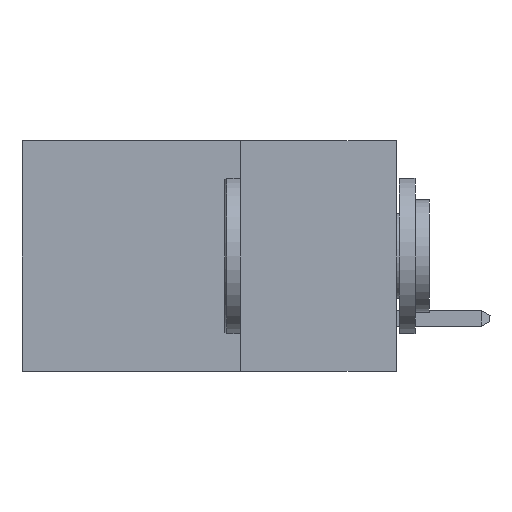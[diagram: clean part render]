
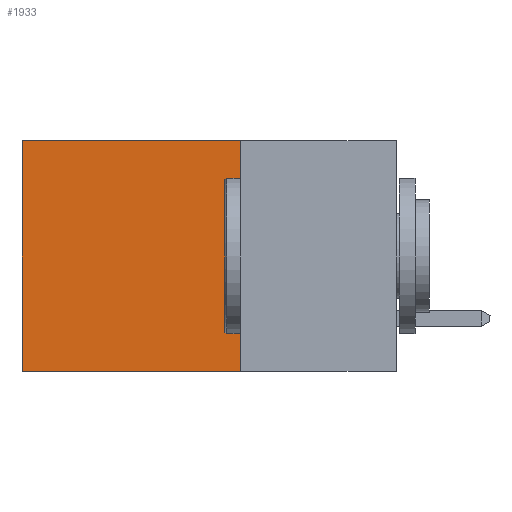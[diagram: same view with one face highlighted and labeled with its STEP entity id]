
A CAD part, left-side view. The second image highlights one B-rep face of the part: STEP entity #1933.
In plain terms, the highlighted planar face has unit normal (-1, 0, 0).
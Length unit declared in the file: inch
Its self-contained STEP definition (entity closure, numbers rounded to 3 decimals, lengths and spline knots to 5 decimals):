
#49 = ORIENTED_EDGE ( 'NONE', *, *, #5225, .F. ) ;
#374 = CARTESIAN_POINT ( 'NONE',  ( 0.2615, 0.25, -0.37 ) ) ;
#1356 = EDGE_CURVE ( 'NONE', #13783, #1747, #13322, .T. ) ;
#1632 = EDGE_CURVE ( 'NONE', #13783, #10384, #12024, .T. ) ;
#1747 = VERTEX_POINT ( 'NONE', #14650 ) ;
#1933 = ADVANCED_FACE ( 'NONE', ( #9175 ), #4695, .F. ) ;
#2579 = DIRECTION ( 'NONE',  ( 0., 0., -1. ) ) ;
#3293 = EDGE_CURVE ( 'NONE', #1747, #7857, #12693, .T. ) ;
#3555 = ORIENTED_EDGE ( 'NONE', *, *, #1356, .T. ) ;
#4169 = CARTESIAN_POINT ( 'NONE',  ( 0.2615, 0.25, -0.37 ) ) ;
#4690 = CARTESIAN_POINT ( 'NONE',  ( 0.2615, 0.6, -0.37 ) ) ;
#4695 = PLANE ( 'NONE',  #12276 ) ;
#4991 = VECTOR ( 'NONE', #2579, 39.37008 ) ;
#5225 = EDGE_CURVE ( 'NONE', #10384, #7857, #10478, .T. ) ;
#6163 = VECTOR ( 'NONE', #7629, 39.37008 ) ;
#7008 = DIRECTION ( 'NONE',  ( 0., 0., -1. ) ) ;
#7010 = CARTESIAN_POINT ( 'NONE',  ( 0.2615, 0.6, -0.37 ) ) ;
#7391 = CARTESIAN_POINT ( 'NONE',  ( 0.2615, 0.25, -0.37 ) ) ;
#7516 = VECTOR ( 'NONE', #10894, 39.37008 ) ;
#7629 = DIRECTION ( 'NONE',  ( 0., 1., 0. ) ) ;
#7857 = VERTEX_POINT ( 'NONE', #4690 ) ;
#7925 = CARTESIAN_POINT ( 'NONE',  ( 0.2615, 0.25, 0. ) ) ;
#8132 = DIRECTION ( 'NONE',  ( 1., 0., 0. ) ) ;
#9175 = FACE_OUTER_BOUND ( 'NONE', #9466, .T. ) ;
#9466 = EDGE_LOOP ( 'NONE', ( #13250, #49, #12880, #3555 ) ) ;
#9510 = DIRECTION ( 'NONE',  ( 0., 1., 0. ) ) ;
#10043 = CARTESIAN_POINT ( 'NONE',  ( 0.2615, 0.25, 0. ) ) ;
#10384 = VERTEX_POINT ( 'NONE', #4169 ) ;
#10478 = LINE ( 'NONE', #374, #14179 ) ;
#10894 = DIRECTION ( 'NONE',  ( 0., 0., -1. ) ) ;
#12024 = LINE ( 'NONE', #7391, #7516 ) ;
#12276 = AXIS2_PLACEMENT_3D ( 'NONE', #14796, #8132, #7008 ) ;
#12693 = LINE ( 'NONE', #7010, #4991 ) ;
#12880 = ORIENTED_EDGE ( 'NONE', *, *, #1632, .F. ) ;
#13250 = ORIENTED_EDGE ( 'NONE', *, *, #3293, .T. ) ;
#13322 = LINE ( 'NONE', #7925, #6163 ) ;
#13783 = VERTEX_POINT ( 'NONE', #10043 ) ;
#14179 = VECTOR ( 'NONE', #9510, 39.37008 ) ;
#14650 = CARTESIAN_POINT ( 'NONE',  ( 0.2615, 0.6, 0. ) ) ;
#14796 = CARTESIAN_POINT ( 'NONE',  ( 0.2615, 0.25, -0.37 ) ) ;
